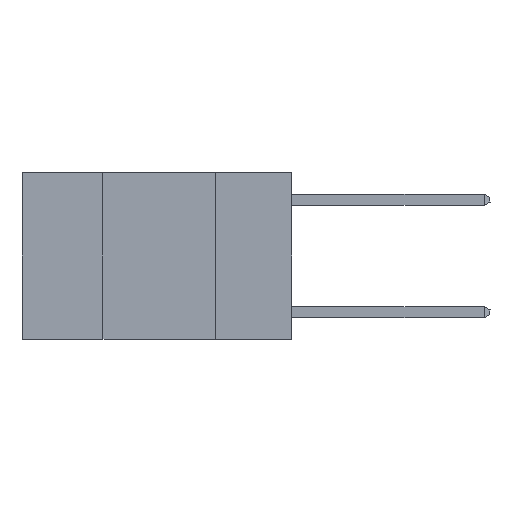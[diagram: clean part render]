
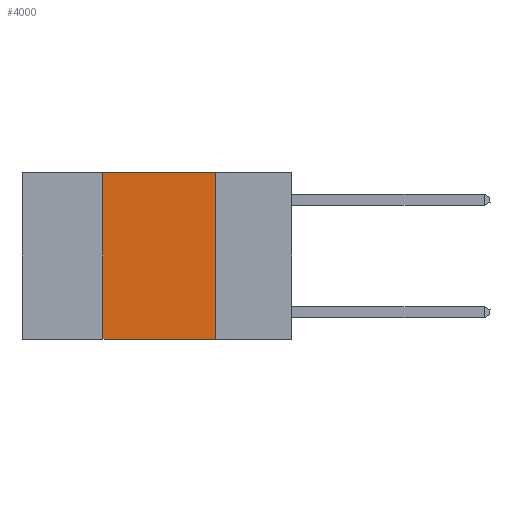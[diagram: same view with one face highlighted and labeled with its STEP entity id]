
A CAD part, left-side view. The second image highlights one B-rep face of the part: STEP entity #4000.
In plain terms, the highlighted planar face has unit normal (-1, 0, 0).
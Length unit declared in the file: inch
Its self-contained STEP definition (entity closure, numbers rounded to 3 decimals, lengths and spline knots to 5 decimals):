
#342 = ORIENTED_EDGE ( 'NONE', *, *, #11460, .F. ) ;
#714 = VERTEX_POINT ( 'NONE', #4064 ) ;
#1729 = EDGE_LOOP ( 'NONE', ( #21875, #342, #15542, #18982 ) ) ;
#2709 = DIRECTION ( 'NONE',  ( 0., 0., -1. ) ) ;
#2931 = VECTOR ( 'NONE', #18438, 39.37008 ) ;
#4000 = ADVANCED_FACE ( 'NONE', ( #25240 ), #12120, .F. ) ;
#4064 = CARTESIAN_POINT ( 'NONE',  ( 0., 0.17, -0.37 ) ) ;
#4403 = CARTESIAN_POINT ( 'NONE',  ( 0., 0.42, -0.37 ) ) ;
#5412 = AXIS2_PLACEMENT_3D ( 'NONE', #24958, #9505, #2709 ) ;
#7755 = CARTESIAN_POINT ( 'NONE',  ( 0., 0.6, -0.37 ) ) ;
#8555 = LINE ( 'NONE', #19835, #20885 ) ;
#9492 = CARTESIAN_POINT ( 'NONE',  ( 0., 0.17, 0. ) ) ;
#9505 = DIRECTION ( 'NONE',  ( 1., 0., 0. ) ) ;
#10945 = LINE ( 'NONE', #19898, #24514 ) ;
#11459 = VERTEX_POINT ( 'NONE', #4403 ) ;
#11460 = EDGE_CURVE ( 'NONE', #15722, #27158, #8555, .T. ) ;
#12100 = EDGE_CURVE ( 'NONE', #11459, #714, #14228, .T. ) ;
#12120 = PLANE ( 'NONE',  #5412 ) ;
#14228 = LINE ( 'NONE', #7755, #18100 ) ;
#15542 = ORIENTED_EDGE ( 'NONE', *, *, #23497, .F. ) ;
#15722 = VERTEX_POINT ( 'NONE', #25989 ) ;
#16716 = DIRECTION ( 'NONE',  ( 0., -1., 0. ) ) ;
#17497 = DIRECTION ( 'NONE',  ( 0., -1., 0. ) ) ;
#18100 = VECTOR ( 'NONE', #16716, 39.37008 ) ;
#18438 = DIRECTION ( 'NONE',  ( 0., 0., -1. ) ) ;
#18982 = ORIENTED_EDGE ( 'NONE', *, *, #12100, .T. ) ;
#19835 = CARTESIAN_POINT ( 'NONE',  ( 0., 0.6, 0. ) ) ;
#19898 = CARTESIAN_POINT ( 'NONE',  ( 0., 0.42, 0. ) ) ;
#20306 = CARTESIAN_POINT ( 'NONE',  ( 0., 0.17, 0. ) ) ;
#20645 = LINE ( 'NONE', #9492, #2931 ) ;
#20885 = VECTOR ( 'NONE', #17497, 39.37008 ) ;
#21875 = ORIENTED_EDGE ( 'NONE', *, *, #25040, .F. ) ;
#22266 = DIRECTION ( 'NONE',  ( 0., 0., 1. ) ) ;
#23497 = EDGE_CURVE ( 'NONE', #11459, #15722, #10945, .T. ) ;
#24514 = VECTOR ( 'NONE', #22266, 39.37008 ) ;
#24958 = CARTESIAN_POINT ( 'NONE',  ( 0., 0.6, 0. ) ) ;
#25040 = EDGE_CURVE ( 'NONE', #27158, #714, #20645, .T. ) ;
#25240 = FACE_OUTER_BOUND ( 'NONE', #1729, .T. ) ;
#25989 = CARTESIAN_POINT ( 'NONE',  ( 0., 0.42, 0. ) ) ;
#27158 = VERTEX_POINT ( 'NONE', #20306 ) ;
